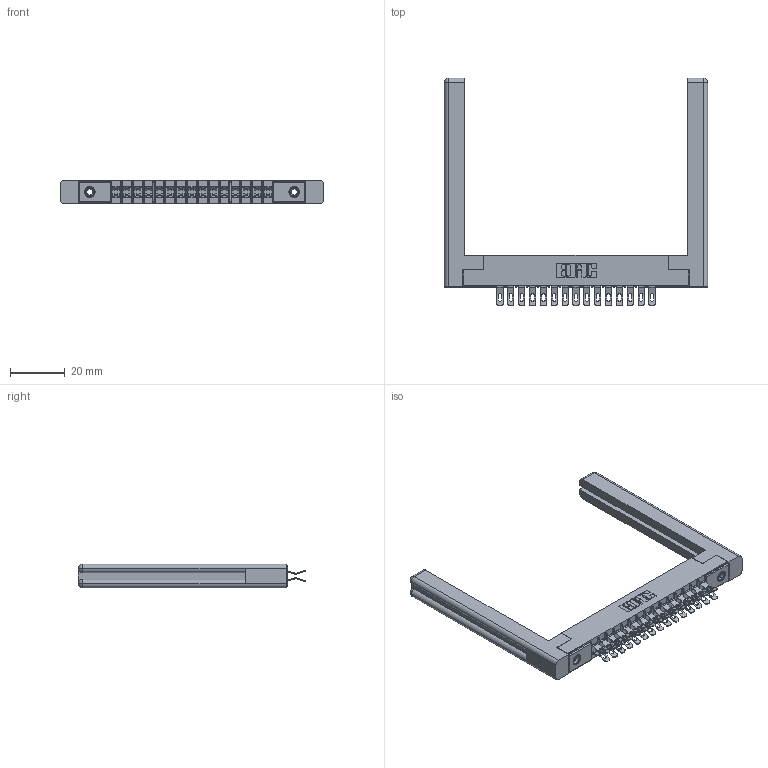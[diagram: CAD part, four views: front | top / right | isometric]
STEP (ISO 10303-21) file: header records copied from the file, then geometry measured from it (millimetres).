
FILE_DESCRIPTION (( 'STEP AP203' ), '1' );
FILE_NAME ('315-030-555-258.STEP', '2019-09-10T15:28:06', ( '' ), ( '' ), 'SwSTEP 2.0', 'SolidWorks 2016', '' );
FILE_SCHEMA (( 'CONFIG_CONTROL_DESIGN' ));
Length unit declared in the file: inch
Products named in the file (5): 305-290-001_555; 307-220-058; 345-250-001_345-250-001-102; 315-030-555-258; 305 Part_.156 Dia
Assembly tree (35 placements, depth 2):
  315-030-555-258
    305 Part_.156 Dia
    305-290-001_555  x30
    345-250-001_345-250-001-102  x2
    307-220-058  x2
Bounding box: 96.06 x 83.06 x 8.71 mm (x, y, z)
Volume: 13851.3 mm3; surface area: 16708.2 mm2
Topology: 35 solids, 35 shells, 2238 faces, 6595 edges, 4302 vertices
Faces by surface type: plane 1112, cylinder 1042, sphere 60, cone 12, torus 12
Entity records: 22785 total; most frequent: CARTESIAN_POINT 3804, ORIENTED_EDGE 3704, DIRECTION 3658, EDGE_CURVE 1852, LINE 1438, VECTOR 1438, VERTEX_POINT 1186, AXIS2_PLACEMENT_3D 1110
